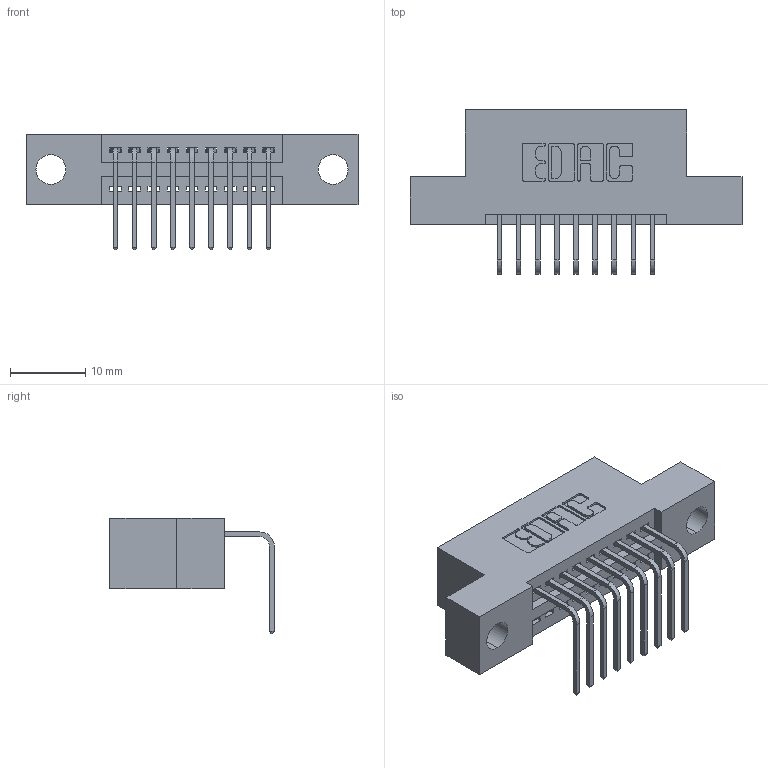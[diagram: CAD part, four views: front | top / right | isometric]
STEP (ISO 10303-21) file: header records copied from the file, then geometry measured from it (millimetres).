
FILE_DESCRIPTION (( 'STEP AP203' ), '1' );
FILE_NAME ('395-009-558-104.STEP', '2021-06-11T13:44:38', ( '' ), ( '' ), 'SwSTEP 2.0', 'SolidWorks 2020', '' );
FILE_SCHEMA (( 'CONFIG_CONTROL_DESIGN' ));
Length unit declared in the file: inch
Products named in the file (3): 395-009-558-104; 345-292-001_558 Tail - 2; 345 Part_Flush Mounting Lugs - 0.156 Dia-TI
Assembly tree (10 placements, depth 2):
  395-009-558-104
    345 Part_Flush Mounting Lugs - 0.156 Dia-TI
    345-292-001_558 Tail - 2  x9
Bounding box: 44.07 x 21.83 x 15.37 mm (x, y, z)
Volume: 3839.4 mm3; surface area: 4672.4 mm2
Topology: 10 solids, 10 shells, 680 faces, 2015 edges, 1330 vertices
Faces by surface type: plane 472, cylinder 208
Entity records: 11719 total; most frequent: CARTESIAN_POINT 2041, ORIENTED_EDGE 1982, DIRECTION 1829, EDGE_CURVE 991, LINE 823, VECTOR 823, VERTEX_POINT 658, AXIS2_PLACEMENT_3D 503
